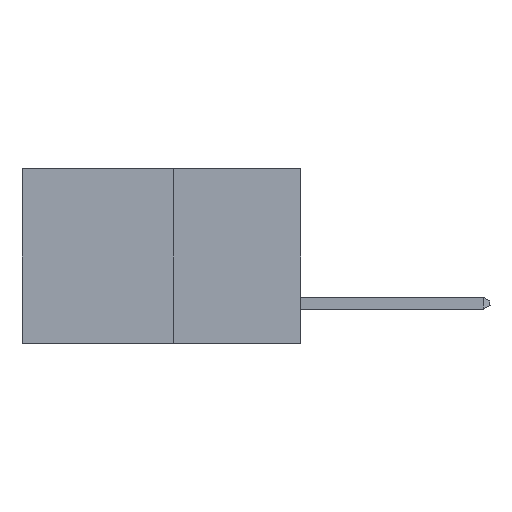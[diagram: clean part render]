
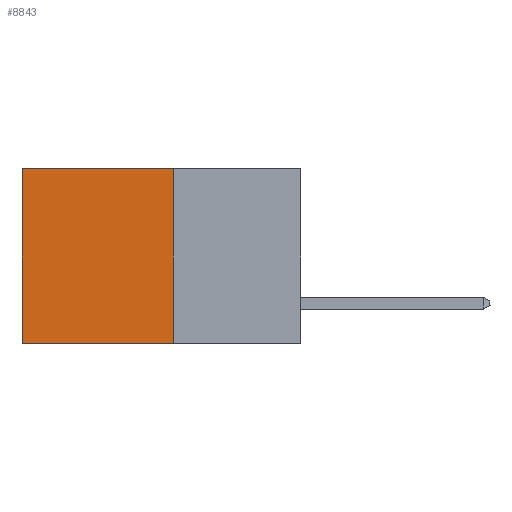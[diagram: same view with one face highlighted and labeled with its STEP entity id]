
A CAD part, left-side view. The second image highlights one B-rep face of the part: STEP entity #8843.
In plain terms, the highlighted planar face has unit normal (-1, 0, 0).
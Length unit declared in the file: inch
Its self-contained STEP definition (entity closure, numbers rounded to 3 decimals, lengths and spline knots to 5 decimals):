
#1476 = LINE ( 'NONE', #6844, #6083 ) ;
#3474 = VECTOR ( 'NONE', #6100, 39.37008 ) ;
#3574 = EDGE_LOOP ( 'NONE', ( #16481, #13777, #17283, #18968 ) ) ;
#4304 = VERTEX_POINT ( 'NONE', #7928 ) ;
#4580 = VERTEX_POINT ( 'NONE', #20450 ) ;
#4814 = LINE ( 'NONE', #21201, #19590 ) ;
#5610 = EDGE_CURVE ( 'NONE', #4304, #16788, #14499, .T. ) ;
#6083 = VECTOR ( 'NONE', #16433, 39.37008 ) ;
#6100 = DIRECTION ( 'NONE',  ( 0., 1., 0. ) ) ;
#6844 = CARTESIAN_POINT ( 'NONE',  ( 0.277, 0.59, -0.37 ) ) ;
#7928 = CARTESIAN_POINT ( 'NONE',  ( 0.277, 0.27, -0.37 ) ) ;
#8223 = DIRECTION ( 'NONE',  ( 0., 0., -1. ) ) ;
#8843 = ADVANCED_FACE ( 'NONE', ( #19095 ), #15850, .F. ) ;
#9494 = CARTESIAN_POINT ( 'NONE',  ( 0.277, 0.27, 0. ) ) ;
#10009 = VECTOR ( 'NONE', #12609, 39.37008 ) ;
#10347 = VERTEX_POINT ( 'NONE', #9494 ) ;
#10674 = CARTESIAN_POINT ( 'NONE',  ( 0.277, 0.27, -0.37 ) ) ;
#12609 = DIRECTION ( 'NONE',  ( 0., 1., 0. ) ) ;
#13617 = EDGE_CURVE ( 'NONE', #4580, #16788, #1476, .T. ) ;
#13777 = ORIENTED_EDGE ( 'NONE', *, *, #5610, .F. ) ;
#14499 = LINE ( 'NONE', #10674, #10009 ) ;
#15628 = CARTESIAN_POINT ( 'NONE',  ( 0.277, 0.59, -0.37 ) ) ;
#15850 = PLANE ( 'NONE',  #21816 ) ;
#15859 = EDGE_CURVE ( 'NONE', #10347, #4304, #4814, .T. ) ;
#16433 = DIRECTION ( 'NONE',  ( 0., 0., -1. ) ) ;
#16481 = ORIENTED_EDGE ( 'NONE', *, *, #13617, .T. ) ;
#16788 = VERTEX_POINT ( 'NONE', #15628 ) ;
#17283 = ORIENTED_EDGE ( 'NONE', *, *, #15859, .F. ) ;
#17788 = CARTESIAN_POINT ( 'NONE',  ( 0.277, 0.27, -0.37 ) ) ;
#18595 = EDGE_CURVE ( 'NONE', #10347, #4580, #18891, .T. ) ;
#18891 = LINE ( 'NONE', #19515, #3474 ) ;
#18968 = ORIENTED_EDGE ( 'NONE', *, *, #18595, .T. ) ;
#19095 = FACE_OUTER_BOUND ( 'NONE', #3574, .T. ) ;
#19515 = CARTESIAN_POINT ( 'NONE',  ( 0.277, 0.27, 0. ) ) ;
#19590 = VECTOR ( 'NONE', #23068, 39.37008 ) ;
#19666 = DIRECTION ( 'NONE',  ( 1., 0., 0. ) ) ;
#20450 = CARTESIAN_POINT ( 'NONE',  ( 0.277, 0.59, 0. ) ) ;
#21201 = CARTESIAN_POINT ( 'NONE',  ( 0.277, 0.27, -0.37 ) ) ;
#21816 = AXIS2_PLACEMENT_3D ( 'NONE', #17788, #19666, #8223 ) ;
#23068 = DIRECTION ( 'NONE',  ( 0., 0., -1. ) ) ;
